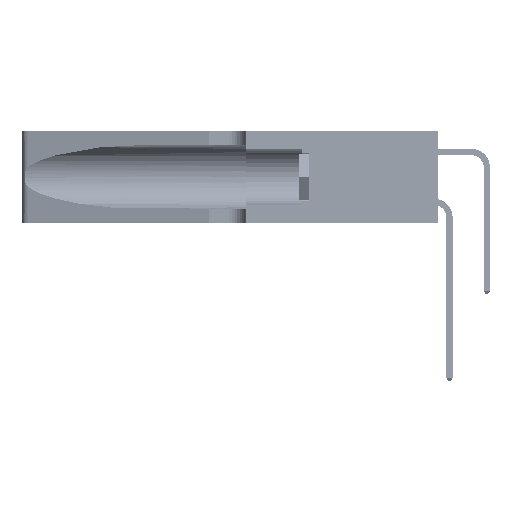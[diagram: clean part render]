
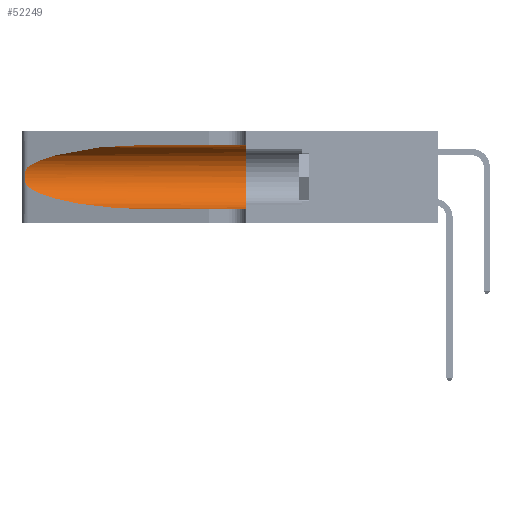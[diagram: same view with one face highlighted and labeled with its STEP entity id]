
A CAD part, left-side view. The second image highlights one B-rep face of the part: STEP entity #52249.
In plain terms, the highlighted cylindrical face has radius 3.308 mm (diameter 6.617 mm), a partial arc.
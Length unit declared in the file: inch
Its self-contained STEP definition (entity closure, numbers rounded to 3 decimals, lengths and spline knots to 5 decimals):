
#2787 = CARTESIAN_POINT ( 'NONE',  ( 0.25487, 1.22718, 0.14631 ) ) ;
#3494 = CARTESIAN_POINT ( 'NONE',  ( 0.26017, 1.23833, 0.17102 ) ) ;
#4604 = CIRCLE ( 'NONE', #39619, 0.13025 ) ;
#4797 = CARTESIAN_POINT ( 'NONE',  ( 0.25487, 1.22718, 0.14631 ) ) ;
#6465 = VECTOR ( 'NONE', #6997, 39.37008 ) ;
#6997 = DIRECTION ( 'NONE',  ( 0., -1., 0. ) ) ;
#7651 = CARTESIAN_POINT ( 'NONE',  ( 0.25789, 1.23486, 0.15765 ) ) ;
#9730 = CYLINDRICAL_SURFACE ( 'NONE', #18274, 0.13025 ) ;
#10965 = VERTEX_POINT ( 'NONE', #52952 ) ;
#11131 = CARTESIAN_POINT ( 'NONE',  ( 0.1305, 0.72297, 0.05475 ) ) ;
#11198 = VECTOR ( 'NONE', #15830, 39.37008 ) ;
#11724 = EDGE_CURVE ( 'NONE', #41873, #10965, #48811, .T. ) ;
#11812 = CARTESIAN_POINT ( 'NONE',  ( 0.25555, 1.22993, 0.14849 ) ) ;
#13003 = CARTESIAN_POINT ( 'NONE',  ( 0.1305, 0.72297, 0.31525 ) ) ;
#13112 = FACE_OUTER_BOUND ( 'NONE', #24700, .T. ) ;
#13662 = CARTESIAN_POINT ( 'NONE',  ( 0.1305, 0.72297, 0.05475 ) ) ;
#15830 = DIRECTION ( 'NONE',  ( 0., -1., 0. ) ) ;
#17175 = CARTESIAN_POINT ( 'NONE',  ( 0.18966, 0.96281, 0.31525 ) ) ;
#17691 = EDGE_CURVE ( 'NONE', #10965, #23027, #29841, .T. ) ;
#18274 = AXIS2_PLACEMENT_3D ( 'NONE', #23078, #27203, #47566 ) ;
#18344 = VERTEX_POINT ( 'NONE', #13662 ) ;
#19848 = EDGE_CURVE ( 'NONE', #41873, #31246, #28441, .T. ) ;
#19950 = CARTESIAN_POINT ( 'NONE',  ( 0.25787, 1.23484, 0.2124 ) ) ;
#20703 = DIRECTION ( 'NONE',  ( 0., 1., 0. ) ) ;
#21324 = CARTESIAN_POINT ( 'NONE',  ( 0.25487, 1.22718, 0.22369 ) ) ;
#21783 = ORIENTED_EDGE ( 'NONE', *, *, #37555, .T. ) ;
#22179 = ORIENTED_EDGE ( 'NONE', *, *, #37449, .T. ) ;
#22194 = LINE ( 'NONE', #44465, #11198 ) ;
#23027 = VERTEX_POINT ( 'NONE', #4797 ) ;
#23078 = CARTESIAN_POINT ( 'NONE',  ( 0.1305, 1.61858, 0.185 ) ) ;
#23735 = CARTESIAN_POINT ( 'NONE',  ( 0.25487, 1.22718, 0.22369 ) ) ;
#23999 = CARTESIAN_POINT ( 'NONE',  ( 0.1305, 0.72297, 0.31525 ) ) ;
#24085 = CARTESIAN_POINT ( 'NONE',  ( 0.26018, 1.23835, 0.19895 ) ) ;
#24700 = EDGE_LOOP ( 'NONE', ( #35051, #32463, #22179, #21783, #51726, #33068 ) ) ;
#27203 = DIRECTION ( 'NONE',  ( 0., -1., 0. ) ) ;
#27545 = CARTESIAN_POINT ( 'NONE',  ( 0.2373, 1.15595, 0.08982 ) ) ;
#28221 = CARTESIAN_POINT ( 'NONE',  ( 0.26075, 1.23896, 0.178 ) ) ;
#28441 = LINE ( 'NONE', #43959, #6465 ) ;
#29841 = B_SPLINE_CURVE_WITH_KNOTS ( 'NONE', 3,
 ( #23735, #40307, #44437, #19950, #48542, #24085, #52631, #28221, #3494, #32331, #7651, #36409, #11812, #40483 ),
 .UNSPECIFIED., .F., .F.,
 ( 4, 2, 2, 2, 2, 2, 4 ),
 ( 0., 0.00027, 0.00053, 0.00107, 0.0016, 0.00187, 0.00214 ),
 .UNSPECIFIED. ) ;
#30402 = EDGE_CURVE ( 'NONE', #31246, #52439, #4604, .T. ) ;
#31246 = VERTEX_POINT ( 'NONE', #42403 ) ;
#32331 = CARTESIAN_POINT ( 'NONE',  ( 0.25856, 1.23593, 0.16098 ) ) ;
#32463 = ORIENTED_EDGE ( 'NONE', *, *, #17691, .T. ) ;
#33068 = ORIENTED_EDGE ( 'NONE', *, *, #19848, .F. ) ;
#35051 = ORIENTED_EDGE ( 'NONE', *, *, #11724, .T. ) ;
#35749 = CARTESIAN_POINT ( 'NONE',  ( 0.18966, 0.96281, 0.05475 ) ) ;
#36409 = CARTESIAN_POINT ( 'NONE',  ( 0.25639, 1.23186, 0.15144 ) ) ;
#37449 = EDGE_CURVE ( 'NONE', #23027, #18344, #50414, .T. ) ;
#37555 = EDGE_CURVE ( 'NONE', #18344, #52439, #22194, .T. ) ;
#39619 = AXIS2_PLACEMENT_3D ( 'NONE', #45180, #20703, #49255 ) ;
#40307 = CARTESIAN_POINT ( 'NONE',  ( 0.25555, 1.22994, 0.2215 ) ) ;
#40483 = CARTESIAN_POINT ( 'NONE',  ( 0.25487, 1.22718, 0.14631 ) ) ;
#41873 = VERTEX_POINT ( 'NONE', #23999 ) ;
#42403 = CARTESIAN_POINT ( 'NONE',  ( 0.1305, 0.35, 0.31525 ) ) ;
#43959 = CARTESIAN_POINT ( 'NONE',  ( 0.1305, 1.61858, 0.31525 ) ) ;
#44437 = CARTESIAN_POINT ( 'NONE',  ( 0.25639, 1.23184, 0.21858 ) ) ;
#44465 = CARTESIAN_POINT ( 'NONE',  ( 0.1305, 1.61858, 0.05475 ) ) ;
#44484 = CARTESIAN_POINT ( 'NONE',  ( 0.1305, 0.35, 0.05475 ) ) ;
#45180 = CARTESIAN_POINT ( 'NONE',  ( 0.1305, 0.35, 0.185 ) ) ;
#45794 = CARTESIAN_POINT ( 'NONE',  ( 0.2373, 1.15595, 0.28018 ) ) ;
#47566 = DIRECTION ( 'NONE',  ( 0., 0., -1. ) ) ;
#48542 = CARTESIAN_POINT ( 'NONE',  ( 0.25854, 1.2359, 0.20912 ) ) ;
#48811 =( BOUNDED_CURVE ( )  B_SPLINE_CURVE ( 3, ( #13003, #17175, #45794, #21324 ),
 .UNSPECIFIED., .F., .F. ) 
 B_SPLINE_CURVE_WITH_KNOTS ( ( 4, 4 ),
 ( 1.5708, 2.84003 ),
 .UNSPECIFIED. ) 
 CURVE ( )  GEOMETRIC_REPRESENTATION_ITEM ( )  RATIONAL_B_SPLINE_CURVE ( ( 1., 0.87, 0.87, 1. ) ) 
 REPRESENTATION_ITEM ( '' )  );
#49255 = DIRECTION ( 'NONE',  ( 0., 0., 1. ) ) ;
#50414 =( BOUNDED_CURVE ( )  B_SPLINE_CURVE ( 3, ( #2787, #27545, #35749, #11131 ),
 .UNSPECIFIED., .F., .F. ) 
 B_SPLINE_CURVE_WITH_KNOTS ( ( 4, 4 ),
 ( 3.44316, 4.71239 ),
 .UNSPECIFIED. ) 
 CURVE ( )  GEOMETRIC_REPRESENTATION_ITEM ( )  RATIONAL_B_SPLINE_CURVE ( ( 1., 0.87, 0.87, 1. ) ) 
 REPRESENTATION_ITEM ( '' )  );
#51726 = ORIENTED_EDGE ( 'NONE', *, *, #30402, .F. ) ;
#52249 = ADVANCED_FACE ( 'NONE', ( #13112 ), #9730, .F. ) ;
#52439 = VERTEX_POINT ( 'NONE', #44484 ) ;
#52631 = CARTESIAN_POINT ( 'NONE',  ( 0.26075, 1.23896, 0.19203 ) ) ;
#52952 = CARTESIAN_POINT ( 'NONE',  ( 0.25487, 1.22718, 0.22369 ) ) ;
